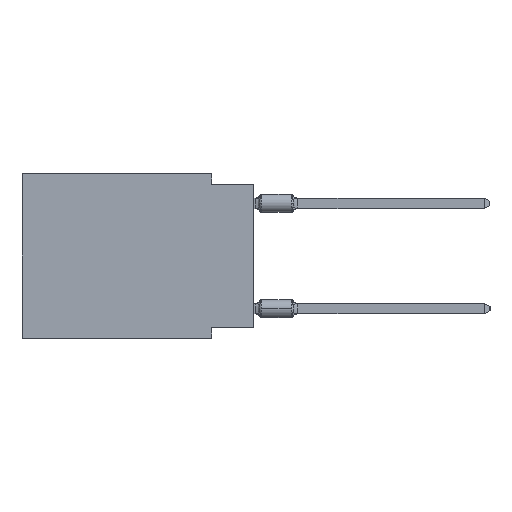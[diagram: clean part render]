
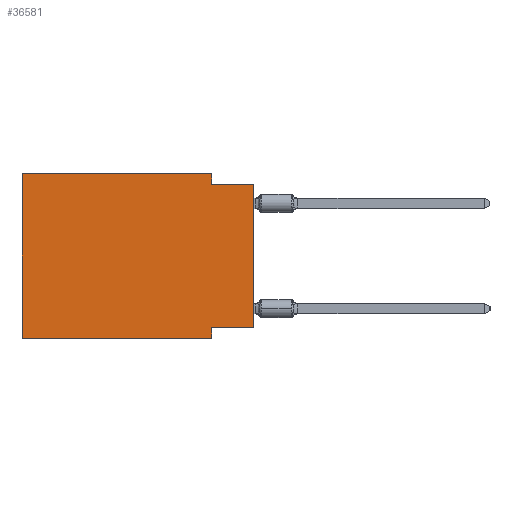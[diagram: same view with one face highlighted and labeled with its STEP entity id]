
A CAD part, left-side view. The second image highlights one B-rep face of the part: STEP entity #36581.
In plain terms, the highlighted planar face has unit normal (-1, 0, 0).
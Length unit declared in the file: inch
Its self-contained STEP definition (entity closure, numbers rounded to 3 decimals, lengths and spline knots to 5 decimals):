
#1 = CARTESIAN_POINT ( 'NONE',  ( 0., 0.55, 0. ) ) ;
#214 = DIRECTION ( 'NONE',  ( 0., -1., 0. ) ) ;
#367 = EDGE_CURVE ( 'NONE', #6574, #32149, #31870, .T. ) ;
#1201 = EDGE_CURVE ( 'NONE', #6574, #20506, #14767, .T. ) ;
#1573 = ORIENTED_EDGE ( 'NONE', *, *, #10244, .F. ) ;
#2224 = EDGE_CURVE ( 'NONE', #32149, #36753, #26783, .T. ) ;
#3248 = ORIENTED_EDGE ( 'NONE', *, *, #17414, .F. ) ;
#3797 = EDGE_CURVE ( 'NONE', #7733, #6279, #15552, .T. ) ;
#4105 = CARTESIAN_POINT ( 'NONE',  ( 0., 0., -0.025 ) ) ;
#5210 = DIRECTION ( 'NONE',  ( 0., -1., 0. ) ) ;
#5716 = ORIENTED_EDGE ( 'NONE', *, *, #2224, .F. ) ;
#5850 = CARTESIAN_POINT ( 'NONE',  ( 0., 0., -0.365 ) ) ;
#6279 = VERTEX_POINT ( 'NONE', #15185 ) ;
#6574 = VERTEX_POINT ( 'NONE', #5850 ) ;
#6803 = ORIENTED_EDGE ( 'NONE', *, *, #367, .F. ) ;
#6814 = CARTESIAN_POINT ( 'NONE',  ( 0., 0.1, 0. ) ) ;
#7733 = VERTEX_POINT ( 'NONE', #8648 ) ;
#8196 = DIRECTION ( 'NONE',  ( 0., 0., -1. ) ) ;
#8578 = DIRECTION ( 'NONE',  ( 0., 1., 0. ) ) ;
#8648 = CARTESIAN_POINT ( 'NONE',  ( 0., 0.55, -0.39 ) ) ;
#9379 = CARTESIAN_POINT ( 'NONE',  ( 0., 0., 0. ) ) ;
#9626 = VERTEX_POINT ( 'NONE', #6814 ) ;
#10005 = DIRECTION ( 'NONE',  ( 0., 0., -1. ) ) ;
#10244 = EDGE_CURVE ( 'NONE', #6279, #9626, #14908, .T. ) ;
#10790 = CARTESIAN_POINT ( 'NONE',  ( 0., 0.1, -0.025 ) ) ;
#11023 = DIRECTION ( 'NONE',  ( 0., -1., 0. ) ) ;
#11692 = AXIS2_PLACEMENT_3D ( 'NONE', #1, #19707, #16906 ) ;
#12225 = EDGE_LOOP ( 'NONE', ( #26302, #3248, #26334, #1573, #29467, #19989, #5716, #6803 ) ) ;
#14136 = CARTESIAN_POINT ( 'NONE',  ( 0., 0.1, 0. ) ) ;
#14346 = VECTOR ( 'NONE', #8578, 39.37008 ) ;
#14564 = VECTOR ( 'NONE', #214, 39.37008 ) ;
#14767 = LINE ( 'NONE', #9379, #19174 ) ;
#14908 = LINE ( 'NONE', #25529, #14564 ) ;
#15185 = CARTESIAN_POINT ( 'NONE',  ( 0., 0.55, 0. ) ) ;
#15552 = LINE ( 'NONE', #18702, #33191 ) ;
#16537 = LINE ( 'NONE', #22304, #21930 ) ;
#16906 = DIRECTION ( 'NONE',  ( 0., 0., -1. ) ) ;
#17414 = EDGE_CURVE ( 'NONE', #18636, #20506, #16537, .T. ) ;
#17673 = CARTESIAN_POINT ( 'NONE',  ( 0., 0., -0.365 ) ) ;
#18391 = CARTESIAN_POINT ( 'NONE',  ( 0., 0.1, -0.39 ) ) ;
#18636 = VERTEX_POINT ( 'NONE', #10790 ) ;
#18702 = CARTESIAN_POINT ( 'NONE',  ( 0., 0.55, 0. ) ) ;
#19174 = VECTOR ( 'NONE', #20159, 39.37008 ) ;
#19707 = DIRECTION ( 'NONE',  ( 1., 0., 0. ) ) ;
#19989 = ORIENTED_EDGE ( 'NONE', *, *, #36056, .T. ) ;
#20159 = DIRECTION ( 'NONE',  ( 0., 0., 1. ) ) ;
#20169 = EDGE_CURVE ( 'NONE', #9626, #18636, #30933, .T. ) ;
#20447 = PLANE ( 'NONE',  #11692 ) ;
#20506 = VERTEX_POINT ( 'NONE', #4105 ) ;
#21568 = CARTESIAN_POINT ( 'NONE',  ( 0., 0.1, -0.365 ) ) ;
#21930 = VECTOR ( 'NONE', #5210, 39.37008 ) ;
#21986 = LINE ( 'NONE', #33393, #33874 ) ;
#22304 = CARTESIAN_POINT ( 'NONE',  ( 0., 0., -0.025 ) ) ;
#25529 = CARTESIAN_POINT ( 'NONE',  ( 0., 0.55, 0. ) ) ;
#26302 = ORIENTED_EDGE ( 'NONE', *, *, #1201, .T. ) ;
#26334 = ORIENTED_EDGE ( 'NONE', *, *, #20169, .F. ) ;
#26783 = LINE ( 'NONE', #27146, #31869 ) ;
#27146 = CARTESIAN_POINT ( 'NONE',  ( 0., 0.1, -0.39 ) ) ;
#29467 = ORIENTED_EDGE ( 'NONE', *, *, #3797, .F. ) ;
#30933 = LINE ( 'NONE', #14136, #34026 ) ;
#31107 = FACE_OUTER_BOUND ( 'NONE', #12225, .T. ) ;
#31869 = VECTOR ( 'NONE', #10005, 39.37008 ) ;
#31870 = LINE ( 'NONE', #17673, #14346 ) ;
#32149 = VERTEX_POINT ( 'NONE', #21568 ) ;
#32888 = DIRECTION ( 'NONE',  ( 0., 0., 1. ) ) ;
#33191 = VECTOR ( 'NONE', #32888, 39.37008 ) ;
#33393 = CARTESIAN_POINT ( 'NONE',  ( 0., 0.55, -0.39 ) ) ;
#33874 = VECTOR ( 'NONE', #11023, 39.37008 ) ;
#34026 = VECTOR ( 'NONE', #8196, 39.37008 ) ;
#36056 = EDGE_CURVE ( 'NONE', #7733, #36753, #21986, .T. ) ;
#36581 = ADVANCED_FACE ( 'NONE', ( #31107 ), #20447, .F. ) ;
#36753 = VERTEX_POINT ( 'NONE', #18391 ) ;
